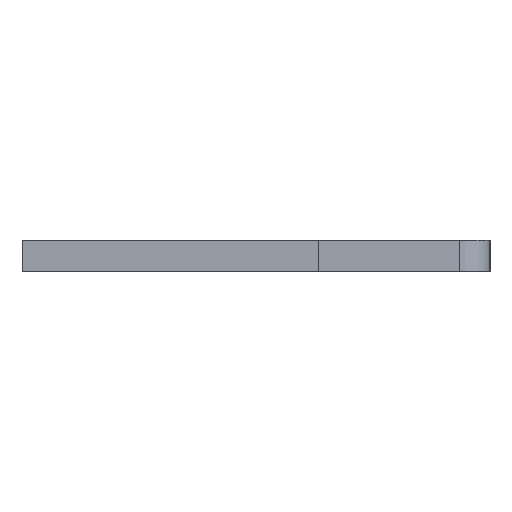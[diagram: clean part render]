
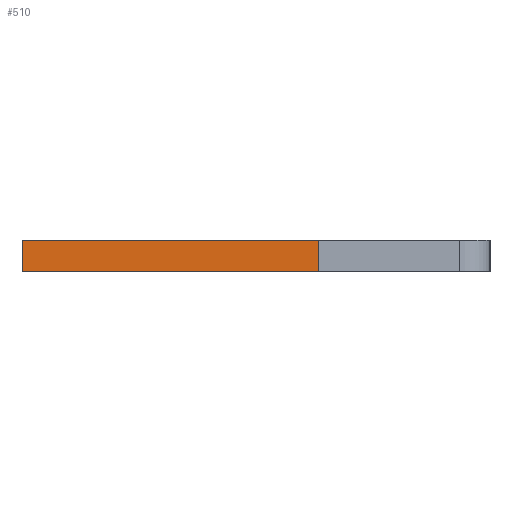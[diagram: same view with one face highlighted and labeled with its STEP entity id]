
A CAD part, left-side view. The second image highlights one B-rep face of the part: STEP entity #510.
In plain terms, the highlighted face is planar.
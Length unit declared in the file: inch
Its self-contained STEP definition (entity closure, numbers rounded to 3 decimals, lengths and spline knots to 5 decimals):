
#69 = ORIENTED_EDGE ( 'NONE', *, *, #1540, .F. ) ;
#73 = VECTOR ( 'NONE', #1144, 39.37008 ) ;
#89 = VERTEX_POINT ( 'NONE', #940 ) ;
#114 = VERTEX_POINT ( 'NONE', #635 ) ;
#131 = PLANE ( 'NONE',  #182 ) ;
#182 = AXIS2_PLACEMENT_3D ( 'NONE', #968, #256, #417 ) ;
#256 = DIRECTION ( 'NONE',  ( 0., 0., 1. ) ) ;
#272 = LINE ( 'NONE', #1367, #418 ) ;
#382 = EDGE_CURVE ( 'NONE', #114, #759, #272, .T. ) ;
#417 = DIRECTION ( 'NONE',  ( 1., 0., 0. ) ) ;
#418 = VECTOR ( 'NONE', #530, 39.37008 ) ;
#510 = ADVANCED_FACE ( 'NONE', ( #617 ), #131, .F. ) ;
#530 = DIRECTION ( 'NONE',  ( -1., 0., 0. ) ) ;
#577 = CARTESIAN_POINT ( 'NONE',  ( -0.01, 0.15, -0.04 ) ) ;
#617 = FACE_OUTER_BOUND ( 'NONE', #1428, .T. ) ;
#635 = CARTESIAN_POINT ( 'NONE',  ( 0.01, 0.15, -0.04 ) ) ;
#722 = DIRECTION ( 'NONE',  ( 0., 1., 0. ) ) ;
#759 = VERTEX_POINT ( 'NONE', #992 ) ;
#803 = ORIENTED_EDGE ( 'NONE', *, *, #979, .T. ) ;
#830 = VERTEX_POINT ( 'NONE', #1125 ) ;
#881 = LINE ( 'NONE', #1419, #73 ) ;
#940 = CARTESIAN_POINT ( 'NONE',  ( -0.01, -0.04, -0.04 ) ) ;
#968 = CARTESIAN_POINT ( 'NONE',  ( 0.01, 0.15, -0.04 ) ) ;
#979 = EDGE_CURVE ( 'NONE', #89, #759, #1560, .T. ) ;
#992 = CARTESIAN_POINT ( 'NONE',  ( -0.01, 0.15, -0.04 ) ) ;
#1125 = CARTESIAN_POINT ( 'NONE',  ( 0.01, -0.04, -0.04 ) ) ;
#1144 = DIRECTION ( 'NONE',  ( -1., 0., 0. ) ) ;
#1165 = CARTESIAN_POINT ( 'NONE',  ( 0.01, 0.15, -0.04 ) ) ;
#1191 = VECTOR ( 'NONE', #1611, 39.37008 ) ;
#1296 = LINE ( 'NONE', #1165, #1191 ) ;
#1339 = EDGE_CURVE ( 'NONE', #830, #89, #881, .T. ) ;
#1367 = CARTESIAN_POINT ( 'NONE',  ( 0.01, 0.15, -0.04 ) ) ;
#1419 = CARTESIAN_POINT ( 'NONE',  ( 0.01, -0.04, -0.04 ) ) ;
#1428 = EDGE_LOOP ( 'NONE', ( #803, #1723, #69, #1470 ) ) ;
#1470 = ORIENTED_EDGE ( 'NONE', *, *, #1339, .T. ) ;
#1489 = VECTOR ( 'NONE', #722, 39.37008 ) ;
#1540 = EDGE_CURVE ( 'NONE', #830, #114, #1296, .T. ) ;
#1560 = LINE ( 'NONE', #577, #1489 ) ;
#1611 = DIRECTION ( 'NONE',  ( 0., 1., 0. ) ) ;
#1723 = ORIENTED_EDGE ( 'NONE', *, *, #382, .F. ) ;
